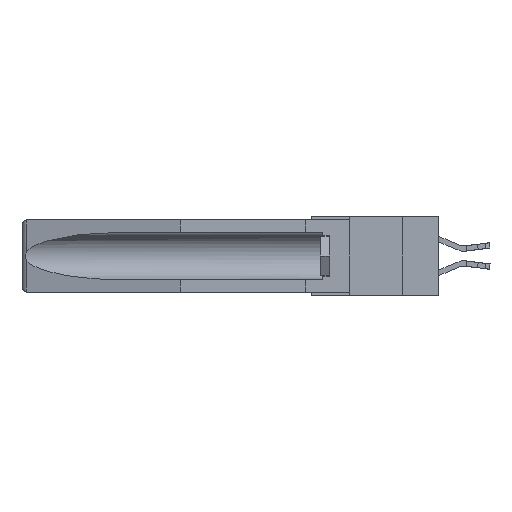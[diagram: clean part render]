
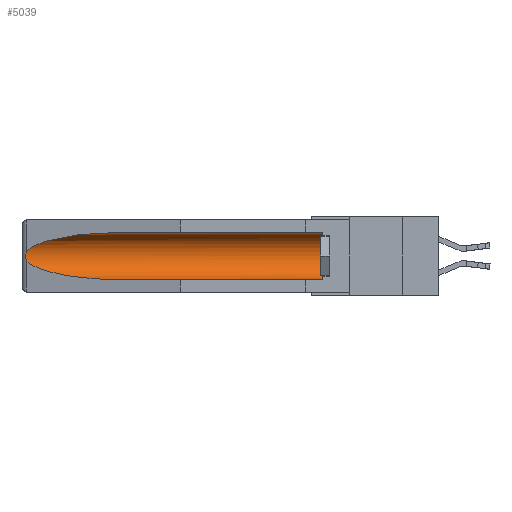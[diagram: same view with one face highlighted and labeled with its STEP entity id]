
A CAD part, left-side view. The second image highlights one B-rep face of the part: STEP entity #5039.
In plain terms, the highlighted cylindrical face has radius 2.857 mm (diameter 5.715 mm), a partial arc.
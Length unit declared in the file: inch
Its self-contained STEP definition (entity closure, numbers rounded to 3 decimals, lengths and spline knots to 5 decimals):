
#656 = EDGE_CURVE ( 'NONE', #7993, #4785, #4965, .T. ) ;
#1637 = CARTESIAN_POINT ( 'NONE',  ( 0.2673, 1.53269, -0.17917 ) ) ;
#1735 = CARTESIAN_POINT ( 'NONE',  ( 0.21114, 1.30732, -0.284 ) ) ;
#1803 = CARTESIAN_POINT ( 'NONE',  ( 0.26537, 1.52718, -0.14972 ) ) ;
#1976 = LINE ( 'NONE', #22331, #22425 ) ;
#2652 = ORIENTED_EDGE ( 'NONE', *, *, #19940, .T. ) ;
#3731 = DIRECTION ( 'NONE',  ( 0., 1., 0. ) ) ;
#4090 = CARTESIAN_POINT ( 'NONE',  ( 0.26537, 1.52718, -0.19328 ) ) ;
#4785 = VERTEX_POINT ( 'NONE', #7047 ) ;
#4949 = FACE_OUTER_BOUND ( 'NONE', #21262, .T. ) ;
#4965 =( BOUNDED_CURVE ( )  B_SPLINE_CURVE ( 3, ( #12377, #21468, #1735, #7118 ),
 .UNSPECIFIED., .F., .F. ) 
 B_SPLINE_CURVE_WITH_KNOTS ( ( 4, 4 ),
 ( 0.1948, 1.5708 ),
 .UNSPECIFIED. ) 
 CURVE ( )  GEOMETRIC_REPRESENTATION_ITEM ( )  RATIONAL_B_SPLINE_CURVE ( ( 1., 0.848, 0.848, 1. ) ) 
 REPRESENTATION_ITEM ( '' )  );
#5039 = ADVANCED_FACE ( 'NONE', ( #4949 ), #18169, .F. ) ;
#5233 = AXIS2_PLACEMENT_3D ( 'NONE', #19498, #19658, #8821 ) ;
#5268 = CARTESIAN_POINT ( 'NONE',  ( 0.26655, 1.53094, -0.18657 ) ) ;
#5907 = CARTESIAN_POINT ( 'NONE',  ( 0.155, 0.126, -0.284 ) ) ;
#7047 = CARTESIAN_POINT ( 'NONE',  ( 0.155, 1.07973, -0.284 ) ) ;
#7118 = CARTESIAN_POINT ( 'NONE',  ( 0.155, 1.07973, -0.284 ) ) ;
#7824 = EDGE_CURVE ( 'NONE', #13891, #9297, #12879, .T. ) ;
#7993 = VERTEX_POINT ( 'NONE', #4090 ) ;
#8298 = CARTESIAN_POINT ( 'NONE',  ( 0.155, 1.07973, -0.059 ) ) ;
#8669 = EDGE_CURVE ( 'NONE', #9297, #18115, #17585, .T. ) ;
#8821 = DIRECTION ( 'NONE',  ( 0., 0., 1. ) ) ;
#8915 = CARTESIAN_POINT ( 'NONE',  ( 0.2675, 1.53308, -0.17534 ) ) ;
#9297 = VERTEX_POINT ( 'NONE', #19196 ) ;
#9379 = CARTESIAN_POINT ( 'NONE',  ( 0.26537, 1.52718, -0.19328 ) ) ;
#9454 = B_SPLINE_CURVE_WITH_KNOTS ( 'NONE', 3,
 ( #1803, #23119, #21460, #16020, #14373, #8915, #1637, #5268, #21394, #9379 ),
 .UNSPECIFIED., .F., .F.,
 ( 4, 2, 2, 2, 4 ),
 ( 0., 0.00029, 0.00058, 0.00087, 0.00117 ),
 .UNSPECIFIED. ) ;
#10126 = CARTESIAN_POINT ( 'NONE',  ( 0.155, 1.07973, -0.059 ) ) ;
#10184 = DIRECTION ( 'NONE',  ( 0., 0., 1. ) ) ;
#11420 = EDGE_CURVE ( 'NONE', #13891, #4785, #1976, .T. ) ;
#11459 = ORIENTED_EDGE ( 'NONE', *, *, #7824, .T. ) ;
#12377 = CARTESIAN_POINT ( 'NONE',  ( 0.26537, 1.52718, -0.19328 ) ) ;
#12879 = CIRCLE ( 'NONE', #20577, 0.1125 ) ;
#13345 = DIRECTION ( 'NONE',  ( 0., 1., 0. ) ) ;
#13656 =( BOUNDED_CURVE ( )  B_SPLINE_CURVE ( 3, ( #8298, #17280, #22471, #18904 ),
 .UNSPECIFIED., .F., .F. ) 
 B_SPLINE_CURVE_WITH_KNOTS ( ( 4, 4 ),
 ( 4.71239, 6.08839 ),
 .UNSPECIFIED. ) 
 CURVE ( )  GEOMETRIC_REPRESENTATION_ITEM ( )  RATIONAL_B_SPLINE_CURVE ( ( 1., 0.848, 0.848, 1. ) ) 
 REPRESENTATION_ITEM ( '' )  );
#13891 = VERTEX_POINT ( 'NONE', #5907 ) ;
#14373 = CARTESIAN_POINT ( 'NONE',  ( 0.2675, 1.53308, -0.16763 ) ) ;
#15577 = CARTESIAN_POINT ( 'NONE',  ( 0.26537, 1.52718, -0.14972 ) ) ;
#16020 = CARTESIAN_POINT ( 'NONE',  ( 0.2673, 1.5327, -0.16383 ) ) ;
#16450 = CARTESIAN_POINT ( 'NONE',  ( 0.155, -0.30754, -0.059 ) ) ;
#16531 = EDGE_CURVE ( 'NONE', #18598, #7993, #9454, .T. ) ;
#16817 = ORIENTED_EDGE ( 'NONE', *, *, #656, .T. ) ;
#17280 = CARTESIAN_POINT ( 'NONE',  ( 0.21114, 1.30732, -0.059 ) ) ;
#17585 = LINE ( 'NONE', #16450, #20352 ) ;
#18115 = VERTEX_POINT ( 'NONE', #10126 ) ;
#18169 = CYLINDRICAL_SURFACE ( 'NONE', #5233, 0.1125 ) ;
#18598 = VERTEX_POINT ( 'NONE', #15577 ) ;
#18841 = CARTESIAN_POINT ( 'NONE',  ( 0.155, 0.126, -0.1715 ) ) ;
#18904 = CARTESIAN_POINT ( 'NONE',  ( 0.26537, 1.52718, -0.14972 ) ) ;
#19196 = CARTESIAN_POINT ( 'NONE',  ( 0.155, 0.126, -0.059 ) ) ;
#19355 = ORIENTED_EDGE ( 'NONE', *, *, #11420, .F. ) ;
#19498 = CARTESIAN_POINT ( 'NONE',  ( 0.155, -0.30754, -0.1715 ) ) ;
#19658 = DIRECTION ( 'NONE',  ( 0., 1., 0. ) ) ;
#19940 = EDGE_CURVE ( 'NONE', #18115, #18598, #13656, .T. ) ;
#20352 = VECTOR ( 'NONE', #3731, 39.37008 ) ;
#20577 = AXIS2_PLACEMENT_3D ( 'NONE', #18841, #20842, #10184 ) ;
#20842 = DIRECTION ( 'NONE',  ( 0., -1., 0. ) ) ;
#21262 = EDGE_LOOP ( 'NONE', ( #2652, #21744, #16817, #19355, #11459, #21946 ) ) ;
#21394 = CARTESIAN_POINT ( 'NONE',  ( 0.26597, 1.5296, -0.19026 ) ) ;
#21460 = CARTESIAN_POINT ( 'NONE',  ( 0.26654, 1.53092, -0.15636 ) ) ;
#21468 = CARTESIAN_POINT ( 'NONE',  ( 0.25451, 1.48313, -0.24835 ) ) ;
#21744 = ORIENTED_EDGE ( 'NONE', *, *, #16531, .T. ) ;
#21946 = ORIENTED_EDGE ( 'NONE', *, *, #8669, .T. ) ;
#22331 = CARTESIAN_POINT ( 'NONE',  ( 0.155, -0.30754, -0.284 ) ) ;
#22425 = VECTOR ( 'NONE', #13345, 39.37008 ) ;
#22471 = CARTESIAN_POINT ( 'NONE',  ( 0.25451, 1.48313, -0.09465 ) ) ;
#23119 = CARTESIAN_POINT ( 'NONE',  ( 0.26597, 1.52961, -0.15275 ) ) ;
